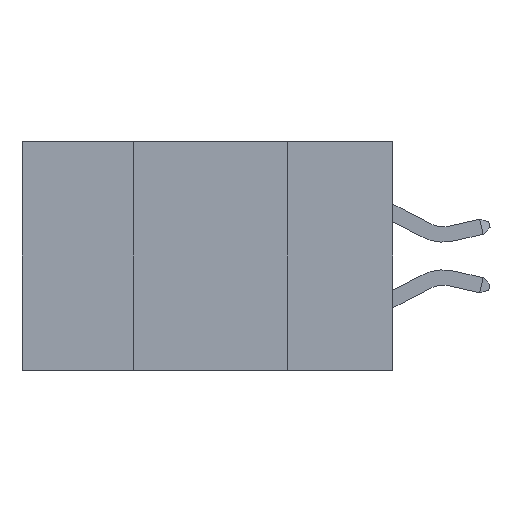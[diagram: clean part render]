
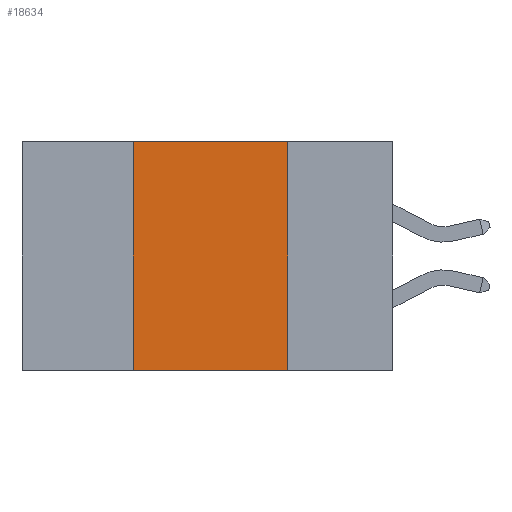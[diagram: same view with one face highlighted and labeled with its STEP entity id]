
A CAD part, left-side view. The second image highlights one B-rep face of the part: STEP entity #18634.
In plain terms, the highlighted planar face has unit normal (-1, 0, 0).
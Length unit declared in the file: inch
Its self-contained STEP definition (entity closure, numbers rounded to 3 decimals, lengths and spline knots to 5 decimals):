
#595 = PLANE ( 'NONE',  #15874 ) ;
#767 = DIRECTION ( 'NONE',  ( 0., -1., 0. ) ) ;
#841 = ORIENTED_EDGE ( 'NONE', *, *, #21866, .T. ) ;
#2194 = CARTESIAN_POINT ( 'NONE',  ( 0., 0.6, -0.37 ) ) ;
#2645 = VERTEX_POINT ( 'NONE', #14780 ) ;
#2974 = VECTOR ( 'NONE', #767, 39.37008 ) ;
#4352 = VECTOR ( 'NONE', #6230, 39.37008 ) ;
#4477 = DIRECTION ( 'NONE',  ( 0., 0., 1. ) ) ;
#4887 = EDGE_CURVE ( 'NONE', #19793, #21207, #14557, .T. ) ;
#5666 = LINE ( 'NONE', #14997, #19273 ) ;
#6230 = DIRECTION ( 'NONE',  ( 0., 0., -1. ) ) ;
#6260 = LINE ( 'NONE', #2194, #7649 ) ;
#7047 = CARTESIAN_POINT ( 'NONE',  ( 0., 0.17, -0.37 ) ) ;
#7649 = VECTOR ( 'NONE', #14531, 39.37008 ) ;
#7902 = CARTESIAN_POINT ( 'NONE',  ( 0., 0.6, 0. ) ) ;
#7997 = CARTESIAN_POINT ( 'NONE',  ( 0., 0.17, 0. ) ) ;
#8056 = EDGE_CURVE ( 'NONE', #21207, #15442, #20197, .T. ) ;
#8697 = ORIENTED_EDGE ( 'NONE', *, *, #14248, .F. ) ;
#10666 = CARTESIAN_POINT ( 'NONE',  ( 0., 0.42, 0. ) ) ;
#11390 = DIRECTION ( 'NONE',  ( 0., 0., -1. ) ) ;
#12916 = CARTESIAN_POINT ( 'NONE',  ( 0., 0.6, 0. ) ) ;
#14248 = EDGE_CURVE ( 'NONE', #2645, #19793, #5666, .T. ) ;
#14531 = DIRECTION ( 'NONE',  ( 0., -1., 0. ) ) ;
#14557 = LINE ( 'NONE', #12916, #2974 ) ;
#14780 = CARTESIAN_POINT ( 'NONE',  ( 0., 0.42, -0.37 ) ) ;
#14997 = CARTESIAN_POINT ( 'NONE',  ( 0., 0.42, 0. ) ) ;
#15442 = VERTEX_POINT ( 'NONE', #7047 ) ;
#15874 = AXIS2_PLACEMENT_3D ( 'NONE', #7902, #22036, #11390 ) ;
#16871 = CARTESIAN_POINT ( 'NONE',  ( 0., 0.17, 0. ) ) ;
#17775 = ORIENTED_EDGE ( 'NONE', *, *, #8056, .F. ) ;
#18634 = ADVANCED_FACE ( 'NONE', ( #21388 ), #595, .F. ) ;
#19071 = EDGE_LOOP ( 'NONE', ( #17775, #19347, #8697, #841 ) ) ;
#19273 = VECTOR ( 'NONE', #4477, 39.37008 ) ;
#19347 = ORIENTED_EDGE ( 'NONE', *, *, #4887, .F. ) ;
#19793 = VERTEX_POINT ( 'NONE', #10666 ) ;
#20197 = LINE ( 'NONE', #16871, #4352 ) ;
#21207 = VERTEX_POINT ( 'NONE', #7997 ) ;
#21388 = FACE_OUTER_BOUND ( 'NONE', #19071, .T. ) ;
#21866 = EDGE_CURVE ( 'NONE', #2645, #15442, #6260, .T. ) ;
#22036 = DIRECTION ( 'NONE',  ( 1., 0., 0. ) ) ;
